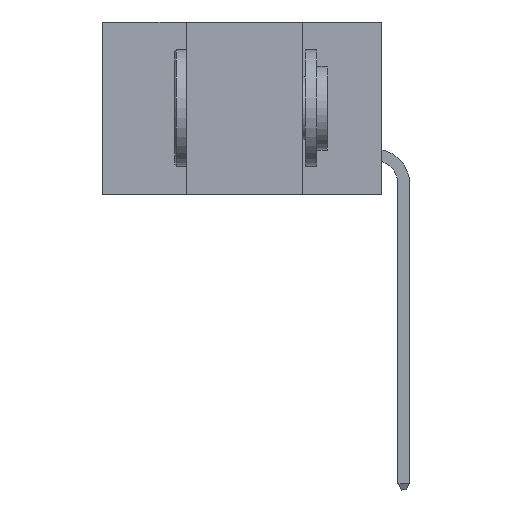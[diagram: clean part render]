
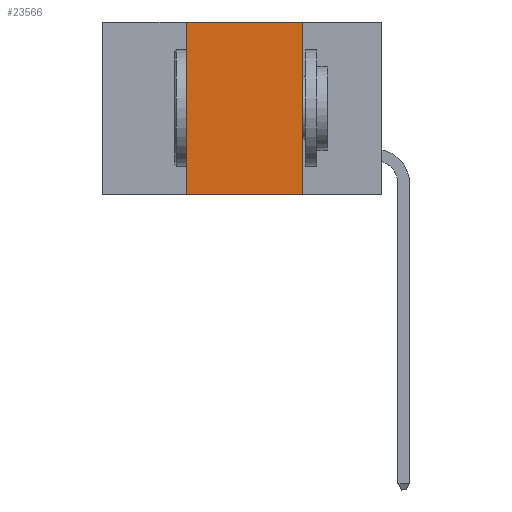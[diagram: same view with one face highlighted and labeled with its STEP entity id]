
A CAD part, left-side view. The second image highlights one B-rep face of the part: STEP entity #23566.
In plain terms, the highlighted planar face has unit normal (-1, 0, 0).
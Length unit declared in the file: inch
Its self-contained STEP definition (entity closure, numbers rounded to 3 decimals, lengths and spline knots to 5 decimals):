
#127 = CARTESIAN_POINT ( 'NONE',  ( 0., 0.6, 0. ) ) ;
#1177 = DIRECTION ( 'NONE',  ( 0., 0., -1. ) ) ;
#1266 = LINE ( 'NONE', #25324, #28307 ) ;
#2274 = CARTESIAN_POINT ( 'NONE',  ( 0., 0.42, -0.37 ) ) ;
#3352 = DIRECTION ( 'NONE',  ( 0., -1., 0. ) ) ;
#7931 = DIRECTION ( 'NONE',  ( 0., 0., 1. ) ) ;
#8158 = CARTESIAN_POINT ( 'NONE',  ( 0., 0.42, 0. ) ) ;
#9379 = LINE ( 'NONE', #37327, #10871 ) ;
#10007 = DIRECTION ( 'NONE',  ( 1., 0., 0. ) ) ;
#10179 = VERTEX_POINT ( 'NONE', #2274 ) ;
#10871 = VECTOR ( 'NONE', #7931, 39.37008 ) ;
#10873 = VERTEX_POINT ( 'NONE', #27182 ) ;
#15129 = AXIS2_PLACEMENT_3D ( 'NONE', #127, #10007, #36092 ) ;
#15652 = EDGE_CURVE ( 'NONE', #10179, #18285, #9379, .T. ) ;
#16608 = VECTOR ( 'NONE', #1177, 39.37008 ) ;
#17488 = EDGE_LOOP ( 'NONE', ( #33920, #37536, #32311, #25817 ) ) ;
#18285 = VERTEX_POINT ( 'NONE', #8158 ) ;
#21551 = VERTEX_POINT ( 'NONE', #35136 ) ;
#22921 = CARTESIAN_POINT ( 'NONE',  ( 0., 0.6, 0. ) ) ;
#23566 = ADVANCED_FACE ( 'NONE', ( #27597 ), #39282, .F. ) ;
#25266 = LINE ( 'NONE', #33983, #16608 ) ;
#25324 = CARTESIAN_POINT ( 'NONE',  ( 0., 0.6, -0.37 ) ) ;
#25817 = ORIENTED_EDGE ( 'NONE', *, *, #42026, .T. ) ;
#26707 = LINE ( 'NONE', #22921, #37997 ) ;
#27182 = CARTESIAN_POINT ( 'NONE',  ( 0., 0.17, 0. ) ) ;
#27597 = FACE_OUTER_BOUND ( 'NONE', #17488, .T. ) ;
#27599 = EDGE_CURVE ( 'NONE', #18285, #10873, #26707, .T. ) ;
#28307 = VECTOR ( 'NONE', #39211, 39.37008 ) ;
#32311 = ORIENTED_EDGE ( 'NONE', *, *, #15652, .F. ) ;
#33920 = ORIENTED_EDGE ( 'NONE', *, *, #38018, .F. ) ;
#33983 = CARTESIAN_POINT ( 'NONE',  ( 0., 0.17, 0. ) ) ;
#35136 = CARTESIAN_POINT ( 'NONE',  ( 0., 0.17, -0.37 ) ) ;
#36092 = DIRECTION ( 'NONE',  ( 0., 0., -1. ) ) ;
#37327 = CARTESIAN_POINT ( 'NONE',  ( 0., 0.42, 0. ) ) ;
#37536 = ORIENTED_EDGE ( 'NONE', *, *, #27599, .F. ) ;
#37997 = VECTOR ( 'NONE', #3352, 39.37008 ) ;
#38018 = EDGE_CURVE ( 'NONE', #10873, #21551, #25266, .T. ) ;
#39211 = DIRECTION ( 'NONE',  ( 0., -1., 0. ) ) ;
#39282 = PLANE ( 'NONE',  #15129 ) ;
#42026 = EDGE_CURVE ( 'NONE', #10179, #21551, #1266, .T. ) ;
